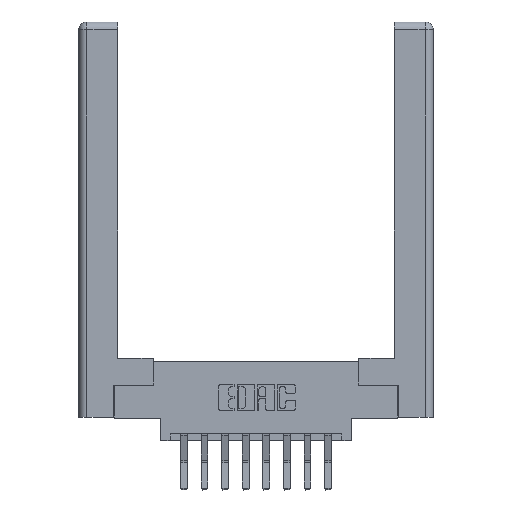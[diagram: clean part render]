
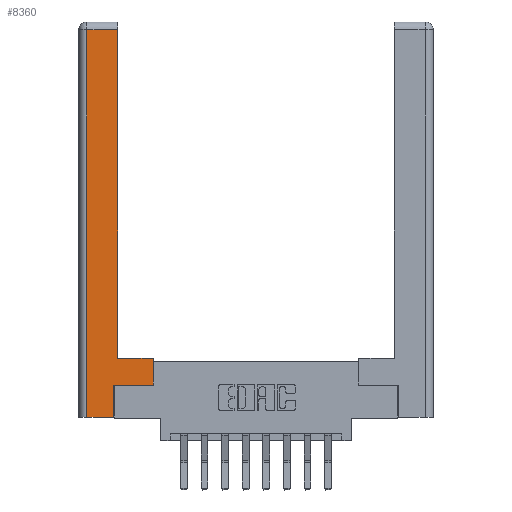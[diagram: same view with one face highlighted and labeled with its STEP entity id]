
A CAD part, top view. The second image highlights one B-rep face of the part: STEP entity #8360.
In plain terms, the highlighted planar face has unit normal (0, 0, 1).
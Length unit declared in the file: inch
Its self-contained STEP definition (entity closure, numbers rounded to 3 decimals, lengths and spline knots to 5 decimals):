
#84 = ORIENTED_EDGE ( 'NONE', *, *, #12406, .T. ) ;
#145 = CARTESIAN_POINT ( 'NONE',  ( 0.565, 0.45, 0. ) ) ;
#157 = LINE ( 'NONE', #2011, #2800 ) ;
#357 = DIRECTION ( 'NONE',  ( -1., 0., 0. ) ) ;
#626 = DIRECTION ( 'NONE',  ( 0., -1., 0. ) ) ;
#937 = DIRECTION ( 'NONE',  ( -1., 0., 0. ) ) ;
#1067 = PLANE ( 'NONE',  #3973 ) ;
#1172 = CARTESIAN_POINT ( 'NONE',  ( 0.565, 0.45, 0. ) ) ;
#1626 = CARTESIAN_POINT ( 'NONE',  ( 0.0615, 2.94, 0. ) ) ;
#1692 = VERTEX_POINT ( 'NONE', #5238 ) ;
#1777 = VERTEX_POINT ( 'NONE', #8265 ) ;
#2011 = CARTESIAN_POINT ( 'NONE',  ( 0.295, 3., 0. ) ) ;
#2114 = VERTEX_POINT ( 'NONE', #9814 ) ;
#2117 = LINE ( 'NONE', #6029, #3902 ) ;
#2239 = LINE ( 'NONE', #11101, #9088 ) ;
#2512 = VECTOR ( 'NONE', #626, 39.37008 ) ;
#2800 = VECTOR ( 'NONE', #12890, 39.37008 ) ;
#2837 = VECTOR ( 'NONE', #5382, 39.37008 ) ;
#3043 = CARTESIAN_POINT ( 'NONE',  ( 0.0615, 0., 0. ) ) ;
#3048 = DIRECTION ( 'NONE',  ( 0., 0., -1. ) ) ;
#3348 = DIRECTION ( 'NONE',  ( 0., 1., 0. ) ) ;
#3544 = CARTESIAN_POINT ( 'NONE',  ( 0.565, 0.245, 0. ) ) ;
#3843 = EDGE_CURVE ( 'NONE', #9777, #2114, #6965, .T. ) ;
#3902 = VECTOR ( 'NONE', #10053, 39.37008 ) ;
#3914 = EDGE_CURVE ( 'NONE', #1777, #4985, #4505, .T. ) ;
#3964 = CARTESIAN_POINT ( 'NONE',  ( 0.295, 2.94, 0. ) ) ;
#3973 = AXIS2_PLACEMENT_3D ( 'NONE', #5101, #3048, #937 ) ;
#4071 = ORIENTED_EDGE ( 'NONE', *, *, #9495, .T. ) ;
#4480 = EDGE_CURVE ( 'NONE', #4985, #9777, #5959, .T. ) ;
#4505 = LINE ( 'NONE', #3544, #12701 ) ;
#4788 = LINE ( 'NONE', #9461, #2837 ) ;
#4985 = VERTEX_POINT ( 'NONE', #10687 ) ;
#5101 = CARTESIAN_POINT ( 'NONE',  ( 0., 0., 0. ) ) ;
#5238 = CARTESIAN_POINT ( 'NONE',  ( 0.265, 0., 0. ) ) ;
#5382 = DIRECTION ( 'NONE',  ( -1., 0., 0. ) ) ;
#5462 = ORIENTED_EDGE ( 'NONE', *, *, #13216, .T. ) ;
#5959 = LINE ( 'NONE', #145, #12588 ) ;
#6029 = CARTESIAN_POINT ( 'NONE',  ( 0.265, 0.245, 0. ) ) ;
#6606 = ORIENTED_EDGE ( 'NONE', *, *, #3843, .T. ) ;
#6746 = EDGE_CURVE ( 'NONE', #2114, #13141, #157, .T. ) ;
#6965 = LINE ( 'NONE', #11144, #7581 ) ;
#7496 = CARTESIAN_POINT ( 'NONE',  ( 0.0615, 0., 0. ) ) ;
#7581 = VECTOR ( 'NONE', #357, 39.37008 ) ;
#7718 = VERTEX_POINT ( 'NONE', #7496 ) ;
#7885 = LINE ( 'NONE', #3043, #2512 ) ;
#8265 = CARTESIAN_POINT ( 'NONE',  ( 0.265, 0.245, 0. ) ) ;
#8360 = ADVANCED_FACE ( 'NONE', ( #9944 ), #1067, .F. ) ;
#8754 = VERTEX_POINT ( 'NONE', #1626 ) ;
#8827 = ORIENTED_EDGE ( 'NONE', *, *, #6746, .T. ) ;
#8831 = ORIENTED_EDGE ( 'NONE', *, *, #3914, .T. ) ;
#9088 = VECTOR ( 'NONE', #12194, 39.37008 ) ;
#9461 = CARTESIAN_POINT ( 'NONE',  ( 0.0615, 2.94, 0. ) ) ;
#9495 = EDGE_CURVE ( 'NONE', #1692, #1777, #2117, .T. ) ;
#9777 = VERTEX_POINT ( 'NONE', #1172 ) ;
#9814 = CARTESIAN_POINT ( 'NONE',  ( 0.295, 0.45, 0. ) ) ;
#9944 = FACE_OUTER_BOUND ( 'NONE', #12689, .T. ) ;
#10053 = DIRECTION ( 'NONE',  ( 0., 1., 0. ) ) ;
#10628 = EDGE_CURVE ( 'NONE', #7718, #1692, #2239, .T. ) ;
#10687 = CARTESIAN_POINT ( 'NONE',  ( 0.565, 0.245, 0. ) ) ;
#11101 = CARTESIAN_POINT ( 'NONE',  ( 0.265, 0., 0. ) ) ;
#11102 = DIRECTION ( 'NONE',  ( 1., 0., 0. ) ) ;
#11144 = CARTESIAN_POINT ( 'NONE',  ( 0.295, 0.45, 0. ) ) ;
#11489 = ORIENTED_EDGE ( 'NONE', *, *, #10628, .T. ) ;
#12138 = ORIENTED_EDGE ( 'NONE', *, *, #4480, .T. ) ;
#12194 = DIRECTION ( 'NONE',  ( 1., 0., 0. ) ) ;
#12406 = EDGE_CURVE ( 'NONE', #8754, #7718, #7885, .T. ) ;
#12588 = VECTOR ( 'NONE', #3348, 39.37008 ) ;
#12689 = EDGE_LOOP ( 'NONE', ( #8827, #5462, #84, #11489, #4071, #8831, #12138, #6606 ) ) ;
#12701 = VECTOR ( 'NONE', #11102, 39.37008 ) ;
#12890 = DIRECTION ( 'NONE',  ( 0., 1., 0. ) ) ;
#13141 = VERTEX_POINT ( 'NONE', #3964 ) ;
#13216 = EDGE_CURVE ( 'NONE', #13141, #8754, #4788, .T. ) ;
